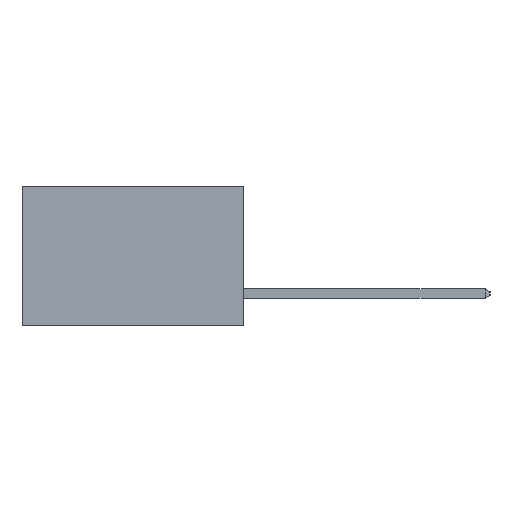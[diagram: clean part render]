
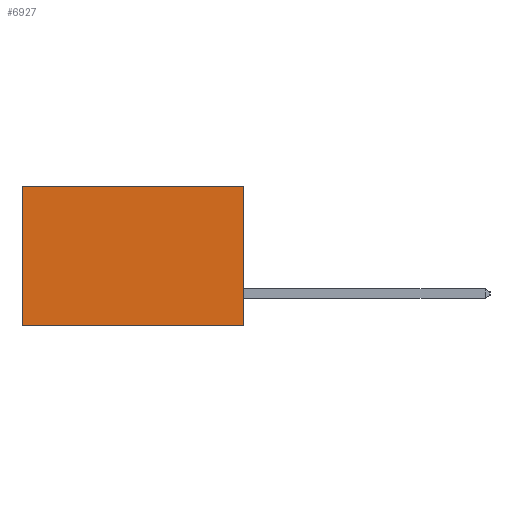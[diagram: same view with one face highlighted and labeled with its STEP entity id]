
A CAD part, left-side view. The second image highlights one B-rep face of the part: STEP entity #6927.
In plain terms, the highlighted planar face has unit normal (-1, 0, 0).
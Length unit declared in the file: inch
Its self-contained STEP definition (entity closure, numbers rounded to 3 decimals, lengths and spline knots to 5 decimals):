
#237 = VERTEX_POINT ( 'NONE', #1024 ) ;
#386 = EDGE_LOOP ( 'NONE', ( #3612, #3935, #6831, #1571 ) ) ;
#752 = VERTEX_POINT ( 'NONE', #6702 ) ;
#1024 = CARTESIAN_POINT ( 'NONE',  ( 0.277, 0.59, 0. ) ) ;
#1571 = ORIENTED_EDGE ( 'NONE', *, *, #11600, .T. ) ;
#1985 = VECTOR ( 'NONE', #4187, 39.37008 ) ;
#2377 = CARTESIAN_POINT ( 'NONE',  ( 0.277, 0.59, -0.37 ) ) ;
#3227 = DIRECTION ( 'NONE',  ( 1., 0., 0. ) ) ;
#3251 = VERTEX_POINT ( 'NONE', #5244 ) ;
#3612 = ORIENTED_EDGE ( 'NONE', *, *, #12775, .T. ) ;
#3935 = ORIENTED_EDGE ( 'NONE', *, *, #7372, .F. ) ;
#4187 = DIRECTION ( 'NONE',  ( 0., 0., -1. ) ) ;
#4227 = VECTOR ( 'NONE', #5818, 39.37008 ) ;
#4243 = FACE_OUTER_BOUND ( 'NONE', #386, .T. ) ;
#4308 = CARTESIAN_POINT ( 'NONE',  ( 0.277, 0., -0.37 ) ) ;
#4565 = EDGE_CURVE ( 'NONE', #11386, #752, #10306, .T. ) ;
#5244 = CARTESIAN_POINT ( 'NONE',  ( 0.277, 0.59, -0.37 ) ) ;
#5370 = PLANE ( 'NONE',  #10954 ) ;
#5818 = DIRECTION ( 'NONE',  ( 0., 1., 0. ) ) ;
#6307 = CARTESIAN_POINT ( 'NONE',  ( 0.277, 0., -0.37 ) ) ;
#6347 = CARTESIAN_POINT ( 'NONE',  ( 0.277, 0., 0. ) ) ;
#6501 = LINE ( 'NONE', #9842, #11792 ) ;
#6702 = CARTESIAN_POINT ( 'NONE',  ( 0.277, 0., -0.37 ) ) ;
#6831 = ORIENTED_EDGE ( 'NONE', *, *, #4565, .F. ) ;
#6927 = ADVANCED_FACE ( 'NONE', ( #4243 ), #5370, .F. ) ;
#6958 = VECTOR ( 'NONE', #7713, 39.37008 ) ;
#7105 = LINE ( 'NONE', #8641, #4227 ) ;
#7372 = EDGE_CURVE ( 'NONE', #752, #3251, #7105, .T. ) ;
#7713 = DIRECTION ( 'NONE',  ( 0., 0., -1. ) ) ;
#7787 = DIRECTION ( 'NONE',  ( 0., 1., 0. ) ) ;
#8641 = CARTESIAN_POINT ( 'NONE',  ( 0.277, 0., -0.37 ) ) ;
#9419 = LINE ( 'NONE', #2377, #6958 ) ;
#9492 = DIRECTION ( 'NONE',  ( 0., 0., -1. ) ) ;
#9842 = CARTESIAN_POINT ( 'NONE',  ( 0.277, 0., 0. ) ) ;
#10306 = LINE ( 'NONE', #4308, #1985 ) ;
#10954 = AXIS2_PLACEMENT_3D ( 'NONE', #6307, #3227, #9492 ) ;
#11386 = VERTEX_POINT ( 'NONE', #6347 ) ;
#11600 = EDGE_CURVE ( 'NONE', #11386, #237, #6501, .T. ) ;
#11792 = VECTOR ( 'NONE', #7787, 39.37008 ) ;
#12775 = EDGE_CURVE ( 'NONE', #237, #3251, #9419, .T. ) ;
